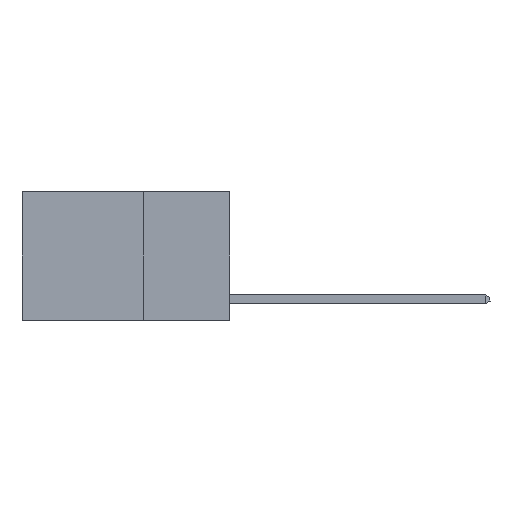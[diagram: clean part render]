
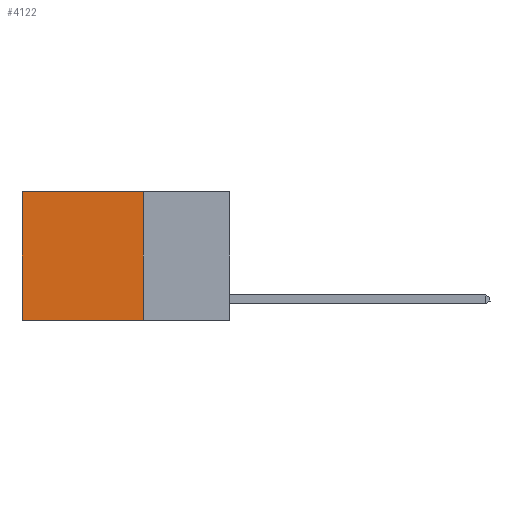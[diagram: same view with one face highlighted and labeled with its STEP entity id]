
A CAD part, left-side view. The second image highlights one B-rep face of the part: STEP entity #4122.
In plain terms, the highlighted planar face has unit normal (-1, 0, 0).
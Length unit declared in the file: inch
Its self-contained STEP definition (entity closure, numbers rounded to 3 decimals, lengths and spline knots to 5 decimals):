
#263 = VECTOR ( 'NONE', #5880, 39.37008 ) ;
#532 = DIRECTION ( 'NONE',  ( 0., 0., -1. ) ) ;
#640 = LINE ( 'NONE', #4754, #263 ) ;
#1033 = CARTESIAN_POINT ( 'NONE',  ( 0.2625, 0.25, 0. ) ) ;
#1236 = ORIENTED_EDGE ( 'NONE', *, *, #13441, .F. ) ;
#1384 = CARTESIAN_POINT ( 'NONE',  ( 0.2625, 0.25, -0.37 ) ) ;
#2069 = VECTOR ( 'NONE', #6740, 39.37008 ) ;
#2903 = EDGE_LOOP ( 'NONE', ( #13887, #1236, #10251, #8249 ) ) ;
#3110 = VERTEX_POINT ( 'NONE', #9773 ) ;
#3587 = VERTEX_POINT ( 'NONE', #12688 ) ;
#4049 = EDGE_CURVE ( 'NONE', #3110, #10607, #640, .T. ) ;
#4122 = ADVANCED_FACE ( 'NONE', ( #8041 ), #12844, .F. ) ;
#4754 = CARTESIAN_POINT ( 'NONE',  ( 0.2625, 0.25, 0. ) ) ;
#4885 = LINE ( 'NONE', #5267, #13346 ) ;
#5267 = CARTESIAN_POINT ( 'NONE',  ( 0.2625, 0.6, 0. ) ) ;
#5880 = DIRECTION ( 'NONE',  ( 0., 1., 0. ) ) ;
#5937 = LINE ( 'NONE', #7044, #9081 ) ;
#6146 = VERTEX_POINT ( 'NONE', #1384 ) ;
#6235 = CARTESIAN_POINT ( 'NONE',  ( 0.2625, 0.25, 0. ) ) ;
#6407 = DIRECTION ( 'NONE',  ( 0., 0., -1. ) ) ;
#6740 = DIRECTION ( 'NONE',  ( 0., 0., -1. ) ) ;
#6844 = CARTESIAN_POINT ( 'NONE',  ( 0.2625, 0.6, 0. ) ) ;
#7044 = CARTESIAN_POINT ( 'NONE',  ( 0.2625, 0.25, -0.37 ) ) ;
#7099 = DIRECTION ( 'NONE',  ( 0., 1., 0. ) ) ;
#7456 = DIRECTION ( 'NONE',  ( 1., 0., 0. ) ) ;
#8041 = FACE_OUTER_BOUND ( 'NONE', #2903, .T. ) ;
#8170 = LINE ( 'NONE', #1033, #2069 ) ;
#8249 = ORIENTED_EDGE ( 'NONE', *, *, #4049, .T. ) ;
#9081 = VECTOR ( 'NONE', #7099, 39.37008 ) ;
#9773 = CARTESIAN_POINT ( 'NONE',  ( 0.2625, 0.25, 0. ) ) ;
#10071 = AXIS2_PLACEMENT_3D ( 'NONE', #6235, #7456, #532 ) ;
#10251 = ORIENTED_EDGE ( 'NONE', *, *, #13230, .F. ) ;
#10607 = VERTEX_POINT ( 'NONE', #6844 ) ;
#12688 = CARTESIAN_POINT ( 'NONE',  ( 0.2625, 0.6, -0.37 ) ) ;
#12844 = PLANE ( 'NONE',  #10071 ) ;
#13027 = EDGE_CURVE ( 'NONE', #10607, #3587, #4885, .T. ) ;
#13230 = EDGE_CURVE ( 'NONE', #3110, #6146, #8170, .T. ) ;
#13346 = VECTOR ( 'NONE', #6407, 39.37008 ) ;
#13441 = EDGE_CURVE ( 'NONE', #6146, #3587, #5937, .T. ) ;
#13887 = ORIENTED_EDGE ( 'NONE', *, *, #13027, .T. ) ;
